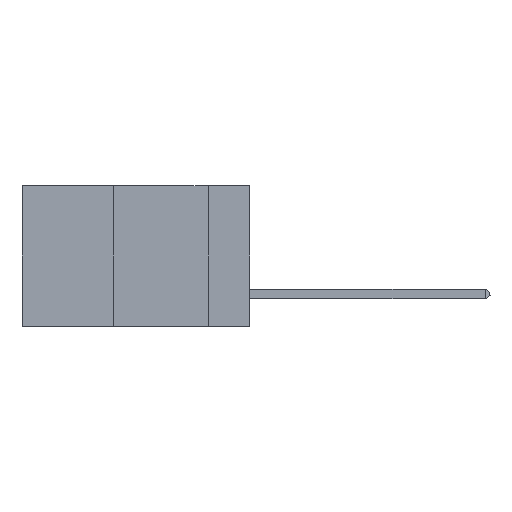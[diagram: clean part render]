
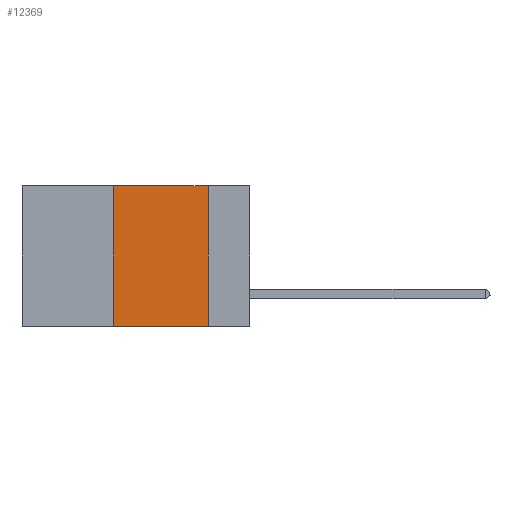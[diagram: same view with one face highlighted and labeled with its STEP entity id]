
A CAD part, left-side view. The second image highlights one B-rep face of the part: STEP entity #12369.
In plain terms, the highlighted planar face has unit normal (-1, 0, 0).
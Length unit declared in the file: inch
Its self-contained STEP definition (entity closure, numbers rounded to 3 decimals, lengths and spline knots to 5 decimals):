
#320 = DIRECTION ( 'NONE',  ( 0., 0., 1. ) ) ;
#530 = LINE ( 'NONE', #13935, #28049 ) ;
#913 = LINE ( 'NONE', #3604, #20100 ) ;
#3604 = CARTESIAN_POINT ( 'NONE',  ( 0., 0.11, 0. ) ) ;
#3814 = DIRECTION ( 'NONE',  ( 0., -1., 0. ) ) ;
#4357 = CARTESIAN_POINT ( 'NONE',  ( 0., 0.11, 0. ) ) ;
#4500 = DIRECTION ( 'NONE',  ( 0., 0., -1. ) ) ;
#5593 = ORIENTED_EDGE ( 'NONE', *, *, #25529, .F. ) ;
#6394 = EDGE_CURVE ( 'NONE', #11560, #23933, #15524, .T. ) ;
#7110 = CARTESIAN_POINT ( 'NONE',  ( 0., 0.36, 0. ) ) ;
#7302 = PLANE ( 'NONE',  #12470 ) ;
#7411 = DIRECTION ( 'NONE',  ( 0., 0., -1. ) ) ;
#7751 = DIRECTION ( 'NONE',  ( 1., 0., 0. ) ) ;
#8343 = ORIENTED_EDGE ( 'NONE', *, *, #16023, .F. ) ;
#9546 = CARTESIAN_POINT ( 'NONE',  ( 0., 0.6, 0. ) ) ;
#11560 = VERTEX_POINT ( 'NONE', #22184 ) ;
#12369 = ADVANCED_FACE ( 'NONE', ( #28402 ), #7302, .F. ) ;
#12470 = AXIS2_PLACEMENT_3D ( 'NONE', #9546, #7751, #7411 ) ;
#12786 = EDGE_CURVE ( 'NONE', #11560, #18064, #18029, .T. ) ;
#13935 = CARTESIAN_POINT ( 'NONE',  ( 0., 0.6, 0. ) ) ;
#15308 = CARTESIAN_POINT ( 'NONE',  ( 0., 0.11, -0.37 ) ) ;
#15524 = LINE ( 'NONE', #16561, #24264 ) ;
#16023 = EDGE_CURVE ( 'NONE', #20732, #18064, #913, .T. ) ;
#16561 = CARTESIAN_POINT ( 'NONE',  ( 0., 0.36, 0. ) ) ;
#18029 = LINE ( 'NONE', #26462, #30754 ) ;
#18064 = VERTEX_POINT ( 'NONE', #15308 ) ;
#19998 = EDGE_LOOP ( 'NONE', ( #8343, #5593, #27118, #26016 ) ) ;
#20100 = VECTOR ( 'NONE', #4500, 39.37008 ) ;
#20732 = VERTEX_POINT ( 'NONE', #4357 ) ;
#22184 = CARTESIAN_POINT ( 'NONE',  ( 0., 0.36, -0.37 ) ) ;
#23933 = VERTEX_POINT ( 'NONE', #7110 ) ;
#24264 = VECTOR ( 'NONE', #320, 39.37008 ) ;
#25529 = EDGE_CURVE ( 'NONE', #23933, #20732, #530, .T. ) ;
#26016 = ORIENTED_EDGE ( 'NONE', *, *, #12786, .T. ) ;
#26462 = CARTESIAN_POINT ( 'NONE',  ( 0., 0.6, -0.37 ) ) ;
#27118 = ORIENTED_EDGE ( 'NONE', *, *, #6394, .F. ) ;
#28049 = VECTOR ( 'NONE', #28938, 39.37008 ) ;
#28402 = FACE_OUTER_BOUND ( 'NONE', #19998, .T. ) ;
#28938 = DIRECTION ( 'NONE',  ( 0., -1., 0. ) ) ;
#30754 = VECTOR ( 'NONE', #3814, 39.37008 ) ;
